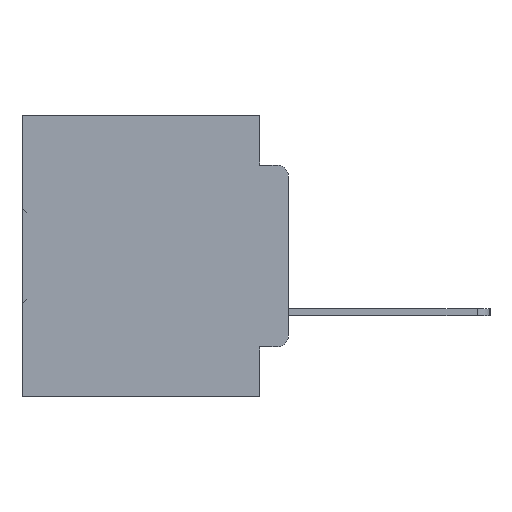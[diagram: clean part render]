
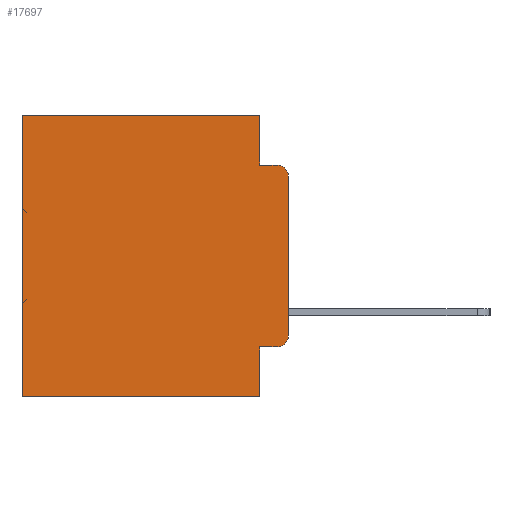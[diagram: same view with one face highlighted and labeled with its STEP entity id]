
A CAD part, left-side view. The second image highlights one B-rep face of the part: STEP entity #17697.
In plain terms, the highlighted planar face has unit normal (-1, 0, 0).
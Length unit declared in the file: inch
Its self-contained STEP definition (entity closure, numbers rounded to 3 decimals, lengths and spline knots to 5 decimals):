
#318 = DIRECTION ( 'NONE',  ( 0., -1., 0. ) ) ;
#821 = CIRCLE ( 'NONE', #17219, 0.02 ) ;
#1334 = ORIENTED_EDGE ( 'NONE', *, *, #26727, .F. ) ;
#2275 = EDGE_CURVE ( 'NONE', #17503, #9564, #14789, .T. ) ;
#2458 = DIRECTION ( 'NONE',  ( 0., 0., -1. ) ) ;
#2679 = VECTOR ( 'NONE', #26125, 39.37008 ) ;
#2776 = EDGE_CURVE ( 'NONE', #31207, #33513, #32153, .T. ) ;
#3967 = EDGE_CURVE ( 'NONE', #16775, #15868, #14659, .T. ) ;
#3982 = CARTESIAN_POINT ( 'NONE',  ( 0.298, 0., 0. ) ) ;
#4071 = DIRECTION ( 'NONE',  ( 0., 0., -1. ) ) ;
#4132 = CARTESIAN_POINT ( 'NONE',  ( 0.298, 0.051, -0.0885 ) ) ;
#5252 = VERTEX_POINT ( 'NONE', #34134 ) ;
#5899 = ORIENTED_EDGE ( 'NONE', *, *, #3967, .F. ) ;
#6099 = VERTEX_POINT ( 'NONE', #19641 ) ;
#6862 = DIRECTION ( 'NONE',  ( 1., 0., 0. ) ) ;
#7086 = VECTOR ( 'NONE', #318, 39.37008 ) ;
#7344 = EDGE_CURVE ( 'NONE', #6099, #18955, #21539, .T. ) ;
#8234 = VECTOR ( 'NONE', #33397, 39.37008 ) ;
#8330 = CARTESIAN_POINT ( 'NONE',  ( 0.298, 0.473, -0.5 ) ) ;
#8583 = EDGE_CURVE ( 'NONE', #32064, #5252, #19113, .T. ) ;
#8806 = VECTOR ( 'NONE', #24127, 39.37008 ) ;
#9359 = CARTESIAN_POINT ( 'NONE',  ( 0.298, 0.051, -0.5 ) ) ;
#9564 = VERTEX_POINT ( 'NONE', #33337 ) ;
#9773 = CARTESIAN_POINT ( 'NONE',  ( 0.298, 0.02, -0.0885 ) ) ;
#10304 = CARTESIAN_POINT ( 'NONE',  ( 0.298, 0.473, 0. ) ) ;
#10720 = ORIENTED_EDGE ( 'NONE', *, *, #8583, .T. ) ;
#10855 = CARTESIAN_POINT ( 'NONE',  ( 0.298, 0.02, -0.3915 ) ) ;
#11175 = ORIENTED_EDGE ( 'NONE', *, *, #21801, .T. ) ;
#12304 = AXIS2_PLACEMENT_3D ( 'NONE', #3982, #6862, #25917 ) ;
#12356 = FACE_OUTER_BOUND ( 'NONE', #12916, .T. ) ;
#12860 = ORIENTED_EDGE ( 'NONE', *, *, #17160, .T. ) ;
#12916 = EDGE_LOOP ( 'NONE', ( #31913, #12860, #20834, #1334, #10720, #34045, #5899, #14122, #30251, #11175 ) ) ;
#12998 = DIRECTION ( 'NONE',  ( 0., -1., 0. ) ) ;
#13587 = DIRECTION ( 'NONE',  ( 0., 0., -1. ) ) ;
#14122 = ORIENTED_EDGE ( 'NONE', *, *, #35118, .F. ) ;
#14355 = CARTESIAN_POINT ( 'NONE',  ( 0.298, 0.02, -0.4115 ) ) ;
#14659 = LINE ( 'NONE', #22560, #8234 ) ;
#14789 = LINE ( 'NONE', #23493, #29593 ) ;
#14889 = VECTOR ( 'NONE', #32612, 39.37008 ) ;
#15403 = CARTESIAN_POINT ( 'NONE',  ( 0.298, 0.051, -0.0885 ) ) ;
#15699 = VECTOR ( 'NONE', #29257, 39.37008 ) ;
#15868 = VERTEX_POINT ( 'NONE', #8330 ) ;
#16775 = VERTEX_POINT ( 'NONE', #9359 ) ;
#17160 = EDGE_CURVE ( 'NONE', #17503, #33513, #821, .T. ) ;
#17219 = AXIS2_PLACEMENT_3D ( 'NONE', #35320, #19023, #2458 ) ;
#17503 = VERTEX_POINT ( 'NONE', #18184 ) ;
#17691 = VECTOR ( 'NONE', #12998, 39.37008 ) ;
#17697 = ADVANCED_FACE ( 'NONE', ( #12356 ), #28507, .F. ) ;
#18184 = CARTESIAN_POINT ( 'NONE',  ( 0.298, 0., -0.1085 ) ) ;
#18392 = CARTESIAN_POINT ( 'NONE',  ( 0.298, 0.051, 0. ) ) ;
#18813 = CARTESIAN_POINT ( 'NONE',  ( 0.298, 0.051, 0. ) ) ;
#18955 = VERTEX_POINT ( 'NONE', #14355 ) ;
#19023 = DIRECTION ( 'NONE',  ( -1., 0., 0. ) ) ;
#19113 = LINE ( 'NONE', #26013, #2679 ) ;
#19641 = CARTESIAN_POINT ( 'NONE',  ( 0.298, 0.051, -0.4115 ) ) ;
#19961 = CIRCLE ( 'NONE', #28947, 0.02 ) ;
#20834 = ORIENTED_EDGE ( 'NONE', *, *, #2776, .F. ) ;
#21539 = LINE ( 'NONE', #25124, #7086 ) ;
#21801 = EDGE_CURVE ( 'NONE', #18955, #9564, #19961, .T. ) ;
#22046 = LINE ( 'NONE', #27121, #14889 ) ;
#22560 = CARTESIAN_POINT ( 'NONE',  ( 0.298, 0., -0.5 ) ) ;
#23493 = CARTESIAN_POINT ( 'NONE',  ( 0.298, 0., 0. ) ) ;
#24127 = DIRECTION ( 'NONE',  ( 0., 0., -1. ) ) ;
#25124 = CARTESIAN_POINT ( 'NONE',  ( 0.298, 0.051, -0.4115 ) ) ;
#25917 = DIRECTION ( 'NONE',  ( 0., 0., -1. ) ) ;
#26013 = CARTESIAN_POINT ( 'NONE',  ( 0.298, 0., 0. ) ) ;
#26125 = DIRECTION ( 'NONE',  ( 0., 1., 0. ) ) ;
#26727 = EDGE_CURVE ( 'NONE', #32064, #31207, #22046, .T. ) ;
#27121 = CARTESIAN_POINT ( 'NONE',  ( 0.298, 0.051, 0. ) ) ;
#27182 = EDGE_CURVE ( 'NONE', #5252, #15868, #27543, .T. ) ;
#27543 = LINE ( 'NONE', #10304, #15699 ) ;
#28507 = PLANE ( 'NONE',  #12304 ) ;
#28947 = AXIS2_PLACEMENT_3D ( 'NONE', #10855, #29818, #13587 ) ;
#29257 = DIRECTION ( 'NONE',  ( 0., 0., -1. ) ) ;
#29593 = VECTOR ( 'NONE', #4071, 39.37008 ) ;
#29818 = DIRECTION ( 'NONE',  ( -1., 0., 0. ) ) ;
#30251 = ORIENTED_EDGE ( 'NONE', *, *, #7344, .T. ) ;
#30506 = LINE ( 'NONE', #18813, #8806 ) ;
#31207 = VERTEX_POINT ( 'NONE', #4132 ) ;
#31913 = ORIENTED_EDGE ( 'NONE', *, *, #2275, .F. ) ;
#32064 = VERTEX_POINT ( 'NONE', #18392 ) ;
#32153 = LINE ( 'NONE', #15403, #17691 ) ;
#32612 = DIRECTION ( 'NONE',  ( 0., 0., -1. ) ) ;
#33337 = CARTESIAN_POINT ( 'NONE',  ( 0.298, 0., -0.3915 ) ) ;
#33397 = DIRECTION ( 'NONE',  ( 0., 1., 0. ) ) ;
#33513 = VERTEX_POINT ( 'NONE', #9773 ) ;
#34045 = ORIENTED_EDGE ( 'NONE', *, *, #27182, .T. ) ;
#34134 = CARTESIAN_POINT ( 'NONE',  ( 0.298, 0.473, 0. ) ) ;
#35118 = EDGE_CURVE ( 'NONE', #6099, #16775, #30506, .T. ) ;
#35320 = CARTESIAN_POINT ( 'NONE',  ( 0.298, 0.02, -0.1085 ) ) ;
